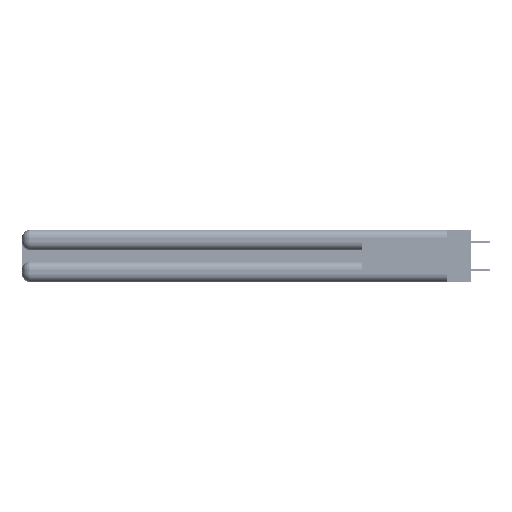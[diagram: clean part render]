
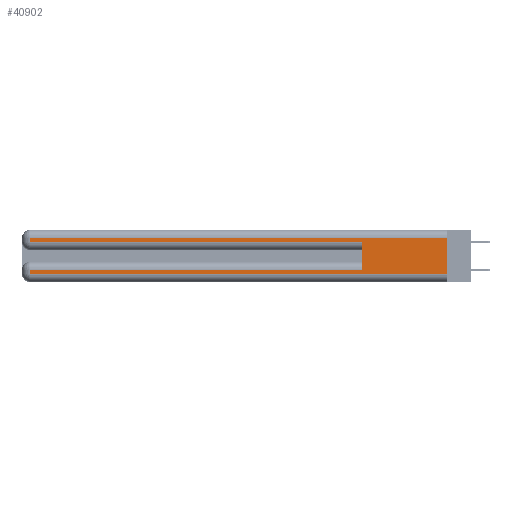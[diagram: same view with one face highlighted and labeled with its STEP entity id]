
A CAD part, left-side view. The second image highlights one B-rep face of the part: STEP entity #40902.
In plain terms, the highlighted planar face has unit normal (-1, 0, 0).
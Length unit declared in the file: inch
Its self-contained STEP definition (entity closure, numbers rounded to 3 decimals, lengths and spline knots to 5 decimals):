
#169 = CARTESIAN_POINT ( 'NONE',  ( 0., 0., 0.31 ) ) ;
#735 = PLANE ( 'NONE',  #23901 ) ;
#2724 = LINE ( 'NONE', #36601, #14945 ) ;
#3260 = ORIENTED_EDGE ( 'NONE', *, *, #26650, .T. ) ;
#3787 = CARTESIAN_POINT ( 'NONE',  ( 0., 0., 0.31 ) ) ;
#4079 = CARTESIAN_POINT ( 'NONE',  ( 0., 0., 0.085 ) ) ;
#4787 = ORIENTED_EDGE ( 'NONE', *, *, #51911, .T. ) ;
#5468 = CARTESIAN_POINT ( 'NONE',  ( 0., 2.94, 0.37 ) ) ;
#6464 = ORIENTED_EDGE ( 'NONE', *, *, #20635, .T. ) ;
#6502 = VERTEX_POINT ( 'NONE', #36974 ) ;
#6536 = ORIENTED_EDGE ( 'NONE', *, *, #39673, .T. ) ;
#7856 = VECTOR ( 'NONE', #49451, 39.37008 ) ;
#9573 = CARTESIAN_POINT ( 'NONE',  ( 0., 2.94, 0.06 ) ) ;
#10047 = DIRECTION ( 'NONE',  ( 0., -1., 0. ) ) ;
#10098 = VERTEX_POINT ( 'NONE', #28546 ) ;
#10554 = DIRECTION ( 'NONE',  ( 0., 0., 1. ) ) ;
#11324 = CARTESIAN_POINT ( 'NONE',  ( 0., 2.94, 0.37 ) ) ;
#12314 = VECTOR ( 'NONE', #50563, 39.37008 ) ;
#12466 = VECTOR ( 'NONE', #10554, 39.37008 ) ;
#13805 = EDGE_CURVE ( 'NONE', #47660, #15508, #35419, .T. ) ;
#14945 = VECTOR ( 'NONE', #48137, 39.37008 ) ;
#15508 = VERTEX_POINT ( 'NONE', #31224 ) ;
#19394 = VECTOR ( 'NONE', #32019, 39.37008 ) ;
#20635 = EDGE_CURVE ( 'NONE', #29351, #44120, #44112, .T. ) ;
#20685 = VECTOR ( 'NONE', #41819, 39.37008 ) ;
#21313 = EDGE_CURVE ( 'NONE', #10098, #15508, #43951, .T. ) ;
#23901 = AXIS2_PLACEMENT_3D ( 'NONE', #50790, #34390, #46957 ) ;
#26029 = ORIENTED_EDGE ( 'NONE', *, *, #21313, .T. ) ;
#26650 = EDGE_CURVE ( 'NONE', #47660, #53856, #34153, .T. ) ;
#28363 = ORIENTED_EDGE ( 'NONE', *, *, #35940, .F. ) ;
#28546 = CARTESIAN_POINT ( 'NONE',  ( 0., 2.94, 0.285 ) ) ;
#29351 = VERTEX_POINT ( 'NONE', #9573 ) ;
#30066 = LINE ( 'NONE', #5468, #12314 ) ;
#31212 = CARTESIAN_POINT ( 'NONE',  ( 0., 0., 0.06 ) ) ;
#31224 = CARTESIAN_POINT ( 'NONE',  ( 0., 0.6, 0.285 ) ) ;
#31273 = CARTESIAN_POINT ( 'NONE',  ( 0., 0.6, 0.145 ) ) ;
#31324 = CARTESIAN_POINT ( 'NONE',  ( 0., 0., 0.285 ) ) ;
#31601 = VECTOR ( 'NONE', #10047, 39.37008 ) ;
#32019 = DIRECTION ( 'NONE',  ( 0., -1., 0. ) ) ;
#34030 = CARTESIAN_POINT ( 'NONE',  ( 0., 2.94, 0.085 ) ) ;
#34153 = LINE ( 'NONE', #4079, #20685 ) ;
#34390 = DIRECTION ( 'NONE',  ( 1., 0., 0. ) ) ;
#34712 = EDGE_CURVE ( 'NONE', #43568, #6502, #45341, .T. ) ;
#35419 = LINE ( 'NONE', #31273, #12466 ) ;
#35940 = EDGE_CURVE ( 'NONE', #43568, #44120, #2724, .T. ) ;
#36601 = CARTESIAN_POINT ( 'NONE',  ( 0., 0., 0.37 ) ) ;
#36974 = CARTESIAN_POINT ( 'NONE',  ( 0., 2.94, 0.31 ) ) ;
#38213 = FACE_OUTER_BOUND ( 'NONE', #45147, .T. ) ;
#39504 = DIRECTION ( 'NONE',  ( 0., 0., -1. ) ) ;
#39636 = ORIENTED_EDGE ( 'NONE', *, *, #34712, .T. ) ;
#39673 = EDGE_CURVE ( 'NONE', #6502, #10098, #43890, .T. ) ;
#40902 = ADVANCED_FACE ( 'NONE', ( #38213 ), #735, .F. ) ;
#41819 = DIRECTION ( 'NONE',  ( 0., 1., 0. ) ) ;
#43568 = VERTEX_POINT ( 'NONE', #169 ) ;
#43890 = LINE ( 'NONE', #11324, #46654 ) ;
#43951 = LINE ( 'NONE', #31324, #31601 ) ;
#44004 = CARTESIAN_POINT ( 'NONE',  ( 0., 0.6, 0.085 ) ) ;
#44112 = LINE ( 'NONE', #31212, #19394 ) ;
#44120 = VERTEX_POINT ( 'NONE', #53031 ) ;
#45147 = EDGE_LOOP ( 'NONE', ( #28363, #39636, #6536, #26029, #48180, #3260, #4787, #6464 ) ) ;
#45341 = LINE ( 'NONE', #3787, #7856 ) ;
#46654 = VECTOR ( 'NONE', #39504, 39.37008 ) ;
#46957 = DIRECTION ( 'NONE',  ( 0., 0., -1. ) ) ;
#47660 = VERTEX_POINT ( 'NONE', #44004 ) ;
#48137 = DIRECTION ( 'NONE',  ( 0., 0., -1. ) ) ;
#48180 = ORIENTED_EDGE ( 'NONE', *, *, #13805, .F. ) ;
#49451 = DIRECTION ( 'NONE',  ( 0., 1., 0. ) ) ;
#50563 = DIRECTION ( 'NONE',  ( 0., 0., -1. ) ) ;
#50790 = CARTESIAN_POINT ( 'NONE',  ( 0., 0., 0.37 ) ) ;
#51911 = EDGE_CURVE ( 'NONE', #53856, #29351, #30066, .T. ) ;
#53031 = CARTESIAN_POINT ( 'NONE',  ( 0., 0., 0.06 ) ) ;
#53856 = VERTEX_POINT ( 'NONE', #34030 ) ;
